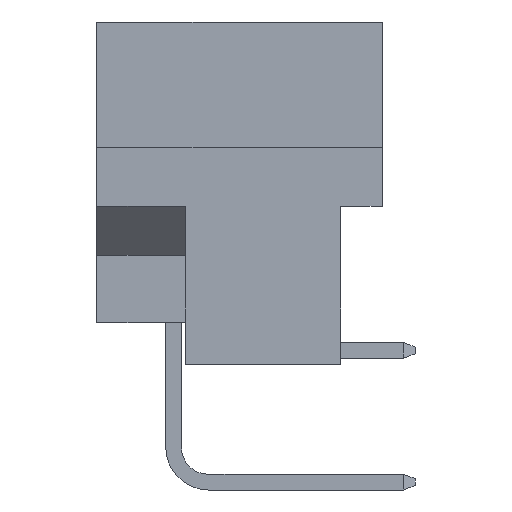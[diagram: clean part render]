
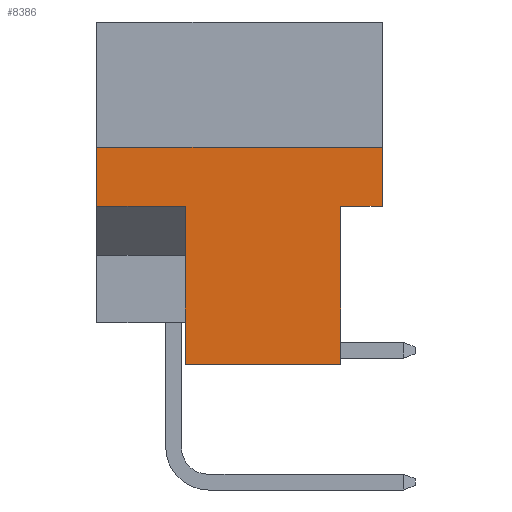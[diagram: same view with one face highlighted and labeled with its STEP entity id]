
A CAD part, left-side view. The second image highlights one B-rep face of the part: STEP entity #8386.
In plain terms, the highlighted planar face has unit normal (-1, 0, 0).
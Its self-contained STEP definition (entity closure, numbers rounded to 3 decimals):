
#985 = VECTOR ( 'NONE', #13840, 1000. ) ;
#1401 = LINE ( 'NONE', #9803, #12773 ) ;
#1485 = DIRECTION ( 'NONE',  ( 0., 0., -1. ) ) ;
#1549 = ORIENTED_EDGE ( 'NONE', *, *, #6768, .T. ) ;
#1762 = CARTESIAN_POINT ( 'NONE',  ( 0., 7.597, -7.112 ) ) ;
#1825 = CARTESIAN_POINT ( 'NONE',  ( 0., 10.998, -7.112 ) ) ;
#1853 = ORIENTED_EDGE ( 'NONE', *, *, #4391, .F. ) ;
#2565 = CARTESIAN_POINT ( 'NONE',  ( 0., 1.6, -7.112 ) ) ;
#2766 = AXIS2_PLACEMENT_3D ( 'NONE', #6467, #11569, #1485 ) ;
#2893 = EDGE_CURVE ( 'NONE', #14495, #5529, #7852, .T. ) ;
#3370 = CARTESIAN_POINT ( 'NONE',  ( 0., 1.6, 86.902 ) ) ;
#4126 = EDGE_CURVE ( 'NONE', #5172, #5719, #7705, .T. ) ;
#4240 = CARTESIAN_POINT ( 'NONE',  ( 0., 10.998, -4.826 ) ) ;
#4367 = ORIENTED_EDGE ( 'NONE', *, *, #4126, .F. ) ;
#4391 = EDGE_CURVE ( 'NONE', #12547, #5172, #1401, .T. ) ;
#4441 = CARTESIAN_POINT ( 'NONE',  ( 0., 7.597, -13.2 ) ) ;
#5044 = EDGE_CURVE ( 'NONE', #15918, #10063, #6499, .T. ) ;
#5172 = VERTEX_POINT ( 'NONE', #1762 ) ;
#5497 = ORIENTED_EDGE ( 'NONE', *, *, #2893, .F. ) ;
#5529 = VERTEX_POINT ( 'NONE', #9881 ) ;
#5627 = LINE ( 'NONE', #3370, #6866 ) ;
#5719 = VERTEX_POINT ( 'NONE', #1825 ) ;
#5811 = VECTOR ( 'NONE', #6330, 1000. ) ;
#6297 = ORIENTED_EDGE ( 'NONE', *, *, #11864, .T. ) ;
#6330 = DIRECTION ( 'NONE',  ( 0., -1., 0. ) ) ;
#6439 = ORIENTED_EDGE ( 'NONE', *, *, #14435, .F. ) ;
#6467 = CARTESIAN_POINT ( 'NONE',  ( 0., 10.998, 0. ) ) ;
#6499 = LINE ( 'NONE', #7962, #6822 ) ;
#6768 = EDGE_CURVE ( 'NONE', #12547, #14132, #15028, .T. ) ;
#6822 = VECTOR ( 'NONE', #7788, 1000. ) ;
#6866 = VECTOR ( 'NONE', #7052, 1000. ) ;
#7052 = DIRECTION ( 'NONE',  ( 0., 0., -1. ) ) ;
#7648 = CARTESIAN_POINT ( 'NONE',  ( 0., 1.6, -13.2 ) ) ;
#7705 = LINE ( 'NONE', #9156, #11217 ) ;
#7788 = DIRECTION ( 'NONE',  ( 0., 1., 0. ) ) ;
#7852 = LINE ( 'NONE', #4240, #985 ) ;
#7962 = CARTESIAN_POINT ( 'NONE',  ( 0., 0., -7.112 ) ) ;
#8386 = ADVANCED_FACE ( 'NONE', ( #10100 ), #10351, .F. ) ;
#8597 = DIRECTION ( 'NONE',  ( 0., 0., 1. ) ) ;
#9069 = CARTESIAN_POINT ( 'NONE',  ( 0., 10.998, -13.2 ) ) ;
#9156 = CARTESIAN_POINT ( 'NONE',  ( 0., 7.597, -7.112 ) ) ;
#9803 = CARTESIAN_POINT ( 'NONE',  ( 0., 7.597, -13.2 ) ) ;
#9881 = CARTESIAN_POINT ( 'NONE',  ( 0., 0., -4.826 ) ) ;
#9894 = CARTESIAN_POINT ( 'NONE',  ( 0., 10.998, 0. ) ) ;
#10063 = VERTEX_POINT ( 'NONE', #2565 ) ;
#10100 = FACE_OUTER_BOUND ( 'NONE', #13479, .T. ) ;
#10351 = PLANE ( 'NONE',  #2766 ) ;
#10453 = DIRECTION ( 'NONE',  ( 0., 1., 0. ) ) ;
#10713 = VECTOR ( 'NONE', #13485, 1000. ) ;
#11000 = LINE ( 'NONE', #14474, #10713 ) ;
#11179 = CARTESIAN_POINT ( 'NONE',  ( 0., 10.998, -4.826 ) ) ;
#11217 = VECTOR ( 'NONE', #10453, 1000. ) ;
#11364 = EDGE_CURVE ( 'NONE', #10063, #14132, #5627, .T. ) ;
#11445 = ORIENTED_EDGE ( 'NONE', *, *, #11364, .F. ) ;
#11516 = CARTESIAN_POINT ( 'NONE',  ( 0., 0., -7.112 ) ) ;
#11569 = DIRECTION ( 'NONE',  ( 1., 0., 0. ) ) ;
#11864 = EDGE_CURVE ( 'NONE', #15918, #5529, #11000, .T. ) ;
#12547 = VERTEX_POINT ( 'NONE', #4441 ) ;
#12773 = VECTOR ( 'NONE', #14786, 1000. ) ;
#13479 = EDGE_LOOP ( 'NONE', ( #11445, #14220, #6297, #5497, #6439, #4367, #1853, #1549 ) ) ;
#13485 = DIRECTION ( 'NONE',  ( 0., 0., 1. ) ) ;
#13612 = LINE ( 'NONE', #9894, #14142 ) ;
#13840 = DIRECTION ( 'NONE',  ( 0., -1., 0. ) ) ;
#14132 = VERTEX_POINT ( 'NONE', #7648 ) ;
#14142 = VECTOR ( 'NONE', #8597, 1000. ) ;
#14220 = ORIENTED_EDGE ( 'NONE', *, *, #5044, .F. ) ;
#14435 = EDGE_CURVE ( 'NONE', #5719, #14495, #13612, .T. ) ;
#14474 = CARTESIAN_POINT ( 'NONE',  ( 0., 0., 0. ) ) ;
#14495 = VERTEX_POINT ( 'NONE', #11179 ) ;
#14786 = DIRECTION ( 'NONE',  ( 0., 0., 1. ) ) ;
#15028 = LINE ( 'NONE', #9069, #5811 ) ;
#15918 = VERTEX_POINT ( 'NONE', #11516 ) ;
